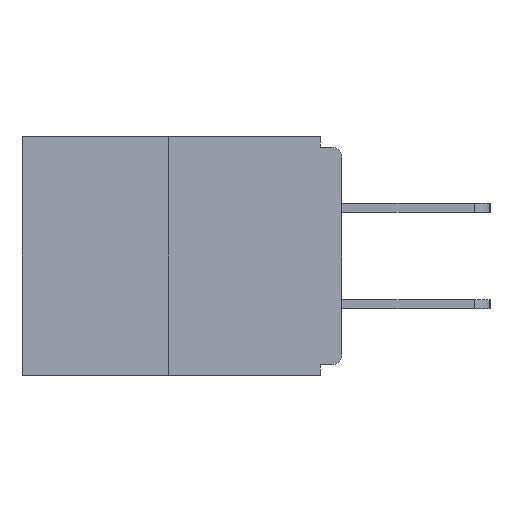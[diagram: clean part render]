
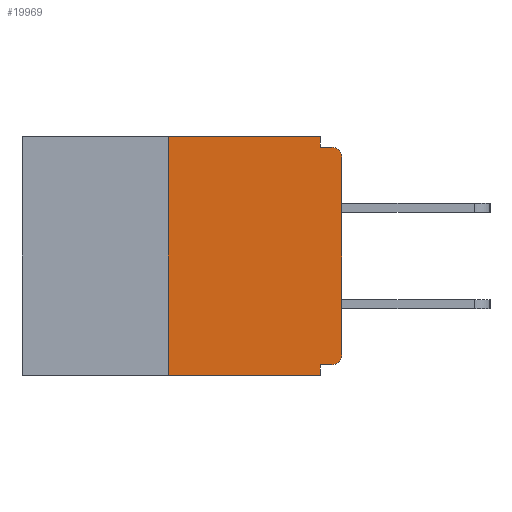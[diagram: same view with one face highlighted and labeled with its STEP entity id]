
A CAD part, left-side view. The second image highlights one B-rep face of the part: STEP entity #19969.
In plain terms, the highlighted planar face has unit normal (-1, 0, 0).
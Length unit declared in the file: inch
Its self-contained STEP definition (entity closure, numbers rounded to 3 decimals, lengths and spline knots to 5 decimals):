
#298 = CARTESIAN_POINT ( 'NONE',  ( 0., 0.46, -0.343 ) ) ;
#622 = EDGE_CURVE ( 'NONE', #18262, #12597, #23956, .T. ) ;
#701 = CARTESIAN_POINT ( 'NONE',  ( 0., 0.031, -0.343 ) ) ;
#1040 = DIRECTION ( 'NONE',  ( 0., 0., -1. ) ) ;
#2079 = DIRECTION ( 'NONE',  ( 0., 0., -1. ) ) ;
#3056 = CARTESIAN_POINT ( 'NONE',  ( 0., 0.031, -0.015 ) ) ;
#3123 = ORIENTED_EDGE ( 'NONE', *, *, #17993, .T. ) ;
#4512 = EDGE_CURVE ( 'NONE', #18124, #17485, #5656, .T. ) ;
#4617 = DIRECTION ( 'NONE',  ( 0., -1., 0. ) ) ;
#4668 = LINE ( 'NONE', #701, #26036 ) ;
#4758 = ORIENTED_EDGE ( 'NONE', *, *, #28486, .F. ) ;
#4793 = LINE ( 'NONE', #7296, #12170 ) ;
#4915 = EDGE_CURVE ( 'NONE', #5841, #27945, #18837, .T. ) ;
#5656 = LINE ( 'NONE', #31801, #10689 ) ;
#5841 = VERTEX_POINT ( 'NONE', #9889 ) ;
#5898 = DIRECTION ( 'NONE',  ( -1., 0., 0. ) ) ;
#6042 = DIRECTION ( 'NONE',  ( 0., 0., -1. ) ) ;
#6151 = CARTESIAN_POINT ( 'NONE',  ( 0., 0., 0. ) ) ;
#6724 = VERTEX_POINT ( 'NONE', #25094 ) ;
#7296 = CARTESIAN_POINT ( 'NONE',  ( 0., 0., -0.015 ) ) ;
#8129 = AXIS2_PLACEMENT_3D ( 'NONE', #10548, #30262, #27887 ) ;
#8378 = DIRECTION ( 'NONE',  ( 0., 0., -1. ) ) ;
#8445 = AXIS2_PLACEMENT_3D ( 'NONE', #20734, #5898, #8378 ) ;
#9039 = CIRCLE ( 'NONE', #8129, 0.015 ) ;
#9889 = CARTESIAN_POINT ( 'NONE',  ( 0., 0.25, -0.343 ) ) ;
#10548 = CARTESIAN_POINT ( 'NONE',  ( 0., 0.015, -0.313 ) ) ;
#10689 = VECTOR ( 'NONE', #4617, 39.37008 ) ;
#10727 = EDGE_CURVE ( 'NONE', #20966, #6724, #21548, .T. ) ;
#11528 = AXIS2_PLACEMENT_3D ( 'NONE', #17025, #29587, #2079 ) ;
#11843 = PLANE ( 'NONE',  #11528 ) ;
#12152 = EDGE_CURVE ( 'NONE', #20447, #6724, #4793, .T. ) ;
#12170 = VECTOR ( 'NONE', #27153, 39.37008 ) ;
#12213 = VECTOR ( 'NONE', #17572, 39.37008 ) ;
#12303 = ORIENTED_EDGE ( 'NONE', *, *, #4915, .T. ) ;
#12563 = ORIENTED_EDGE ( 'NONE', *, *, #622, .F. ) ;
#12597 = VERTEX_POINT ( 'NONE', #12971 ) ;
#12787 = EDGE_CURVE ( 'NONE', #5841, #18124, #20660, .T. ) ;
#12971 = CARTESIAN_POINT ( 'NONE',  ( 0., 0.031, -0.328 ) ) ;
#14320 = CARTESIAN_POINT ( 'NONE',  ( 0., 0.015, -0.328 ) ) ;
#14336 = FACE_OUTER_BOUND ( 'NONE', #17530, .T. ) ;
#14377 = ORIENTED_EDGE ( 'NONE', *, *, #10727, .T. ) ;
#14648 = ORIENTED_EDGE ( 'NONE', *, *, #19184, .F. ) ;
#14699 = VECTOR ( 'NONE', #30717, 39.37008 ) ;
#15723 = CARTESIAN_POINT ( 'NONE',  ( 0., 0.25, 0. ) ) ;
#16471 = CARTESIAN_POINT ( 'NONE',  ( 0., 0.25, 0. ) ) ;
#16706 = ORIENTED_EDGE ( 'NONE', *, *, #4512, .F. ) ;
#16932 = VECTOR ( 'NONE', #25994, 39.37008 ) ;
#17025 = CARTESIAN_POINT ( 'NONE',  ( 0., 0.46, 0. ) ) ;
#17485 = VERTEX_POINT ( 'NONE', #27224 ) ;
#17530 = EDGE_LOOP ( 'NONE', ( #16706, #26159, #12303, #14648, #12563, #3123, #21673, #14377, #23794, #4758 ) ) ;
#17572 = DIRECTION ( 'NONE',  ( 0., -1., 0. ) ) ;
#17993 = EDGE_CURVE ( 'NONE', #18262, #19391, #9039, .T. ) ;
#18124 = VERTEX_POINT ( 'NONE', #15723 ) ;
#18262 = VERTEX_POINT ( 'NONE', #14320 ) ;
#18837 = LINE ( 'NONE', #298, #12213 ) ;
#19184 = EDGE_CURVE ( 'NONE', #12597, #27945, #4668, .T. ) ;
#19391 = VERTEX_POINT ( 'NONE', #21938 ) ;
#19969 = ADVANCED_FACE ( 'NONE', ( #14336 ), #11843, .F. ) ;
#20447 = VERTEX_POINT ( 'NONE', #3056 ) ;
#20660 = LINE ( 'NONE', #16471, #28819 ) ;
#20734 = CARTESIAN_POINT ( 'NONE',  ( 0., 0.015, -0.03 ) ) ;
#20966 = VERTEX_POINT ( 'NONE', #29548 ) ;
#21439 = CARTESIAN_POINT ( 'NONE',  ( 0., 0.031, -0.343 ) ) ;
#21548 = CIRCLE ( 'NONE', #8445, 0.015 ) ;
#21666 = DIRECTION ( 'NONE',  ( 0., 0., 1. ) ) ;
#21673 = ORIENTED_EDGE ( 'NONE', *, *, #28423, .T. ) ;
#21696 = LINE ( 'NONE', #28452, #23200 ) ;
#21938 = CARTESIAN_POINT ( 'NONE',  ( 0., 0., -0.313 ) ) ;
#23200 = VECTOR ( 'NONE', #6042, 39.37008 ) ;
#23794 = ORIENTED_EDGE ( 'NONE', *, *, #12152, .F. ) ;
#23915 = CARTESIAN_POINT ( 'NONE',  ( 0., 0., -0.328 ) ) ;
#23956 = LINE ( 'NONE', #23915, #16932 ) ;
#25094 = CARTESIAN_POINT ( 'NONE',  ( 0., 0.015, -0.015 ) ) ;
#25608 = LINE ( 'NONE', #6151, #14699 ) ;
#25994 = DIRECTION ( 'NONE',  ( 0., 1., 0. ) ) ;
#26036 = VECTOR ( 'NONE', #1040, 39.37008 ) ;
#26159 = ORIENTED_EDGE ( 'NONE', *, *, #12787, .F. ) ;
#27153 = DIRECTION ( 'NONE',  ( 0., -1., 0. ) ) ;
#27224 = CARTESIAN_POINT ( 'NONE',  ( 0., 0.031, 0. ) ) ;
#27887 = DIRECTION ( 'NONE',  ( 0., 0., -1. ) ) ;
#27945 = VERTEX_POINT ( 'NONE', #21439 ) ;
#28423 = EDGE_CURVE ( 'NONE', #19391, #20966, #25608, .T. ) ;
#28452 = CARTESIAN_POINT ( 'NONE',  ( 0., 0.031, 0. ) ) ;
#28486 = EDGE_CURVE ( 'NONE', #17485, #20447, #21696, .T. ) ;
#28819 = VECTOR ( 'NONE', #21666, 39.37008 ) ;
#29548 = CARTESIAN_POINT ( 'NONE',  ( 0., 0., -0.03 ) ) ;
#29587 = DIRECTION ( 'NONE',  ( 1., 0., 0. ) ) ;
#30262 = DIRECTION ( 'NONE',  ( -1., 0., 0. ) ) ;
#30717 = DIRECTION ( 'NONE',  ( 0., 0., 1. ) ) ;
#31801 = CARTESIAN_POINT ( 'NONE',  ( 0., 0.46, 0. ) ) ;
